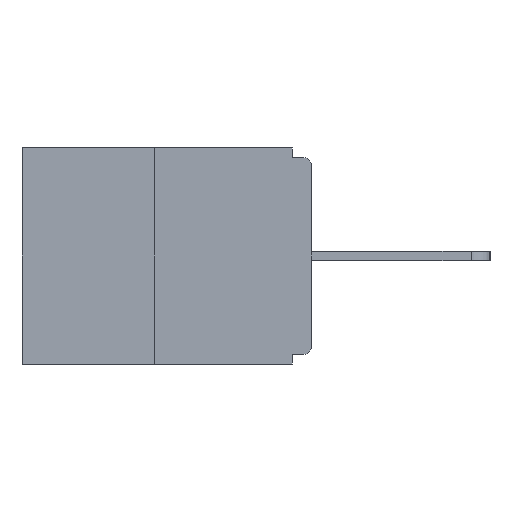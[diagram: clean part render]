
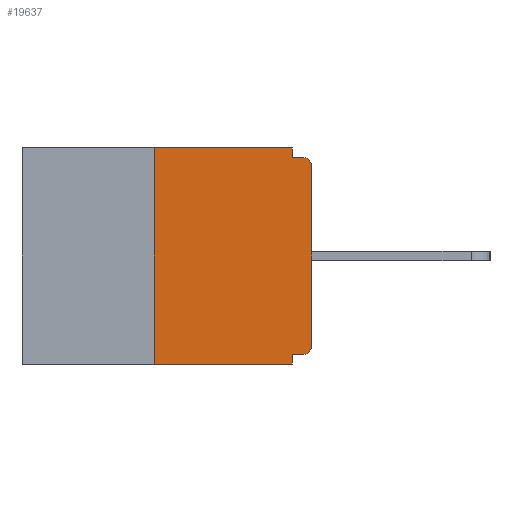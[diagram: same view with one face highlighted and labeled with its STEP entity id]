
A CAD part, left-side view. The second image highlights one B-rep face of the part: STEP entity #19637.
In plain terms, the highlighted planar face has unit normal (-1, 0, 0).
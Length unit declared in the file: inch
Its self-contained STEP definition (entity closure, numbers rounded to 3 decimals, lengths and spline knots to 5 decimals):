
#69 = VERTEX_POINT ( 'NONE', #7368 ) ;
#156 = VECTOR ( 'NONE', #22753, 39.37008 ) ;
#1470 = VERTEX_POINT ( 'NONE', #20265 ) ;
#1644 = CARTESIAN_POINT ( 'NONE',  ( 0., 0., -0.015 ) ) ;
#1883 = CARTESIAN_POINT ( 'NONE',  ( 0., 0.46, 0. ) ) ;
#1993 = VERTEX_POINT ( 'NONE', #22515 ) ;
#2807 = DIRECTION ( 'NONE',  ( 1., 0., 0. ) ) ;
#3601 = CARTESIAN_POINT ( 'NONE',  ( 0., 0.25, -0.343 ) ) ;
#3769 = DIRECTION ( 'NONE',  ( 0., 0., -1. ) ) ;
#4093 = AXIS2_PLACEMENT_3D ( 'NONE', #21065, #5188, #12255 ) ;
#4234 = LINE ( 'NONE', #13011, #21596 ) ;
#4972 = CARTESIAN_POINT ( 'NONE',  ( 0., 0.031, 0. ) ) ;
#5188 = DIRECTION ( 'NONE',  ( -1., 0., 0. ) ) ;
#5460 = DIRECTION ( 'NONE',  ( 0., -1., 0. ) ) ;
#5758 = VECTOR ( 'NONE', #5460, 39.37008 ) ;
#5936 = DIRECTION ( 'NONE',  ( 0., -1., 0. ) ) ;
#6006 = AXIS2_PLACEMENT_3D ( 'NONE', #21900, #2807, #15167 ) ;
#6417 = ORIENTED_EDGE ( 'NONE', *, *, #12166, .T. ) ;
#6665 = ORIENTED_EDGE ( 'NONE', *, *, #20356, .F. ) ;
#6730 = CARTESIAN_POINT ( 'NONE',  ( 0., 0., -0.313 ) ) ;
#7057 = DIRECTION ( 'NONE',  ( 0., -1., 0. ) ) ;
#7343 = VECTOR ( 'NONE', #21382, 39.37008 ) ;
#7368 = CARTESIAN_POINT ( 'NONE',  ( 0., 0.25, 0. ) ) ;
#7899 = CARTESIAN_POINT ( 'NONE',  ( 0., 0.46, -0.343 ) ) ;
#7924 = ORIENTED_EDGE ( 'NONE', *, *, #22445, .F. ) ;
#8070 = VECTOR ( 'NONE', #18785, 39.37008 ) ;
#8344 = VERTEX_POINT ( 'NONE', #12550 ) ;
#8596 = EDGE_CURVE ( 'NONE', #10383, #1470, #9649, .T. ) ;
#8656 = DIRECTION ( 'NONE',  ( 0., 0., -1. ) ) ;
#8751 = EDGE_CURVE ( 'NONE', #10383, #69, #13678, .T. ) ;
#8983 = CARTESIAN_POINT ( 'NONE',  ( 0., 0., -0.03 ) ) ;
#9649 = LINE ( 'NONE', #7899, #18435 ) ;
#9755 = ORIENTED_EDGE ( 'NONE', *, *, #8751, .F. ) ;
#9847 = VERTEX_POINT ( 'NONE', #10108 ) ;
#9942 = CARTESIAN_POINT ( 'NONE',  ( 0., 0.031, -0.328 ) ) ;
#10108 = CARTESIAN_POINT ( 'NONE',  ( 0., 0.031, 0. ) ) ;
#10139 = AXIS2_PLACEMENT_3D ( 'NONE', #14054, #21022, #3769 ) ;
#10324 = ORIENTED_EDGE ( 'NONE', *, *, #11697, .F. ) ;
#10383 = VERTEX_POINT ( 'NONE', #3601 ) ;
#10840 = EDGE_CURVE ( 'NONE', #22334, #12745, #16155, .T. ) ;
#11156 = VECTOR ( 'NONE', #8656, 39.37008 ) ;
#11697 = EDGE_CURVE ( 'NONE', #1993, #8344, #14014, .T. ) ;
#12013 = CARTESIAN_POINT ( 'NONE',  ( 0., 0.015, -0.328 ) ) ;
#12035 = CARTESIAN_POINT ( 'NONE',  ( 0., 0., 0. ) ) ;
#12166 = EDGE_CURVE ( 'NONE', #12482, #22334, #20729, .T. ) ;
#12255 = DIRECTION ( 'NONE',  ( 0., 0., -1. ) ) ;
#12482 = VERTEX_POINT ( 'NONE', #12013 ) ;
#12550 = CARTESIAN_POINT ( 'NONE',  ( 0., 0.015, -0.015 ) ) ;
#12745 = VERTEX_POINT ( 'NONE', #8983 ) ;
#13011 = CARTESIAN_POINT ( 'NONE',  ( 0., 0., -0.328 ) ) ;
#13387 = EDGE_CURVE ( 'NONE', #9847, #1993, #19092, .T. ) ;
#13453 = CARTESIAN_POINT ( 'NONE',  ( 0., 0.25, 0. ) ) ;
#13591 = VERTEX_POINT ( 'NONE', #9942 ) ;
#13678 = LINE ( 'NONE', #13453, #8070 ) ;
#14014 = LINE ( 'NONE', #1644, #21072 ) ;
#14054 = CARTESIAN_POINT ( 'NONE',  ( 0., 0.015, -0.03 ) ) ;
#14793 = ORIENTED_EDGE ( 'NONE', *, *, #20824, .F. ) ;
#14899 = ORIENTED_EDGE ( 'NONE', *, *, #13387, .F. ) ;
#15167 = DIRECTION ( 'NONE',  ( 0., 0., -1. ) ) ;
#15676 = CARTESIAN_POINT ( 'NONE',  ( 0., 0.031, -0.343 ) ) ;
#16109 = LINE ( 'NONE', #1883, #5758 ) ;
#16155 = LINE ( 'NONE', #12035, #7343 ) ;
#16908 = FACE_OUTER_BOUND ( 'NONE', #20523, .T. ) ;
#16941 = ORIENTED_EDGE ( 'NONE', *, *, #10840, .T. ) ;
#17149 = ORIENTED_EDGE ( 'NONE', *, *, #20781, .T. ) ;
#17423 = LINE ( 'NONE', #15676, #156 ) ;
#18435 = VECTOR ( 'NONE', #5936, 39.37008 ) ;
#18785 = DIRECTION ( 'NONE',  ( 0., 0., 1. ) ) ;
#19092 = LINE ( 'NONE', #4972, #11156 ) ;
#19637 = ADVANCED_FACE ( 'NONE', ( #16908 ), #21790, .F. ) ;
#20085 = DIRECTION ( 'NONE',  ( 0., 1., 0. ) ) ;
#20122 = CIRCLE ( 'NONE', #10139, 0.015 ) ;
#20265 = CARTESIAN_POINT ( 'NONE',  ( 0., 0.031, -0.343 ) ) ;
#20356 = EDGE_CURVE ( 'NONE', #12482, #13591, #4234, .T. ) ;
#20523 = EDGE_LOOP ( 'NONE', ( #7924, #9755, #20767, #14793, #6665, #6417, #16941, #17149, #10324, #14899 ) ) ;
#20729 = CIRCLE ( 'NONE', #4093, 0.015 ) ;
#20767 = ORIENTED_EDGE ( 'NONE', *, *, #8596, .T. ) ;
#20781 = EDGE_CURVE ( 'NONE', #12745, #8344, #20122, .T. ) ;
#20824 = EDGE_CURVE ( 'NONE', #13591, #1470, #17423, .T. ) ;
#21022 = DIRECTION ( 'NONE',  ( -1., 0., 0. ) ) ;
#21065 = CARTESIAN_POINT ( 'NONE',  ( 0., 0.015, -0.313 ) ) ;
#21072 = VECTOR ( 'NONE', #7057, 39.37008 ) ;
#21382 = DIRECTION ( 'NONE',  ( 0., 0., 1. ) ) ;
#21596 = VECTOR ( 'NONE', #20085, 39.37008 ) ;
#21790 = PLANE ( 'NONE',  #6006 ) ;
#21900 = CARTESIAN_POINT ( 'NONE',  ( 0., 0.46, 0. ) ) ;
#22334 = VERTEX_POINT ( 'NONE', #6730 ) ;
#22445 = EDGE_CURVE ( 'NONE', #69, #9847, #16109, .T. ) ;
#22515 = CARTESIAN_POINT ( 'NONE',  ( 0., 0.031, -0.015 ) ) ;
#22753 = DIRECTION ( 'NONE',  ( 0., 0., -1. ) ) ;
